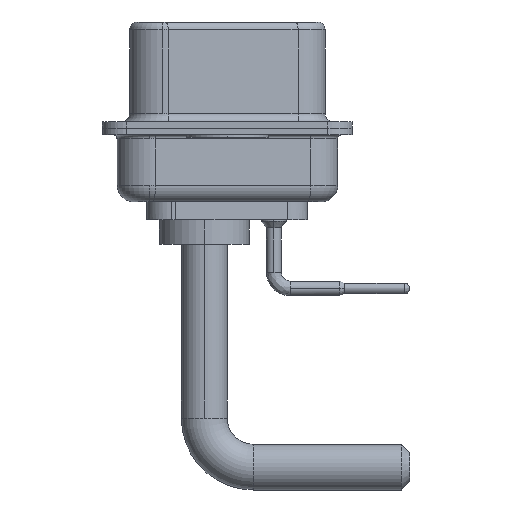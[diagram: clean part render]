
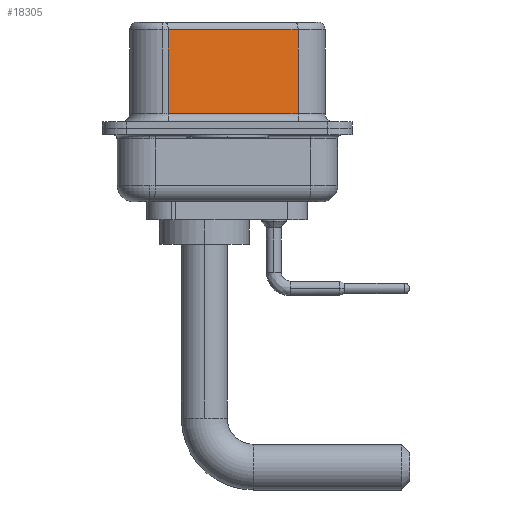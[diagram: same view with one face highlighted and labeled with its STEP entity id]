
A CAD part, left-side view. The second image highlights one B-rep face of the part: STEP entity #18305.
In plain terms, the highlighted planar face has unit normal (-0.985, -0.174, 0).
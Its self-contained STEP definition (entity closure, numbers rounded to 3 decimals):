
#445 = LINE ( 'NONE', #21000, #8310 ) ;
#653 = VERTEX_POINT ( 'NONE', #3463 ) ;
#831 = LINE ( 'NONE', #14577, #10171 ) ;
#2503 = EDGE_CURVE ( 'NONE', #653, #12462, #831, .T. ) ;
#3463 = CARTESIAN_POINT ( 'NONE',  ( 3.73, 3.628, 6.02 ) ) ;
#4261 = VECTOR ( 'NONE', #22033, 1000. ) ;
#5703 = ORIENTED_EDGE ( 'NONE', *, *, #13592, .F. ) ;
#5996 = VECTOR ( 'NONE', #9553, 1000. ) ;
#6199 = CARTESIAN_POINT ( 'NONE',  ( 5.132, -4.322, 6.52 ) ) ;
#6239 = VERTEX_POINT ( 'NONE', #21685 ) ;
#6333 = EDGE_LOOP ( 'NONE', ( #5703, #16460, #7844, #14801 ) ) ;
#6748 = CARTESIAN_POINT ( 'NONE',  ( 5.132, -4.322, 6.02 ) ) ;
#7844 = ORIENTED_EDGE ( 'NONE', *, *, #2503, .T. ) ;
#8310 = VECTOR ( 'NONE', #21101, 1000. ) ;
#9550 = VERTEX_POINT ( 'NONE', #12229 ) ;
#9553 = DIRECTION ( 'NONE',  ( 0., 0., -1. ) ) ;
#9778 = DIRECTION ( 'NONE',  ( -0.174, 0.985, 0. ) ) ;
#10171 = VECTOR ( 'NONE', #19817, 1000. ) ;
#10180 = LINE ( 'NONE', #6748, #4261 ) ;
#11218 = CARTESIAN_POINT ( 'NONE',  ( 5.132, -4.322, 6.52 ) ) ;
#11450 = FACE_OUTER_BOUND ( 'NONE', #6333, .T. ) ;
#12229 = CARTESIAN_POINT ( 'NONE',  ( 5.132, -4.322, 0.9 ) ) ;
#12462 = VERTEX_POINT ( 'NONE', #18582 ) ;
#13592 = EDGE_CURVE ( 'NONE', #6239, #9550, #21484, .T. ) ;
#14278 = DIRECTION ( 'NONE',  ( 0.985, 0.174, 0. ) ) ;
#14577 = CARTESIAN_POINT ( 'NONE',  ( 3.73, 3.628, 6.52 ) ) ;
#14612 = AXIS2_PLACEMENT_3D ( 'NONE', #11218, #14278, #9778 ) ;
#14801 = ORIENTED_EDGE ( 'NONE', *, *, #20710, .T. ) ;
#14916 = PLANE ( 'NONE',  #14612 ) ;
#16460 = ORIENTED_EDGE ( 'NONE', *, *, #17484, .T. ) ;
#17484 = EDGE_CURVE ( 'NONE', #6239, #653, #10180, .T. ) ;
#18305 = ADVANCED_FACE ( 'NONE', ( #11450 ), #14916, .F. ) ;
#18582 = CARTESIAN_POINT ( 'NONE',  ( 3.73, 3.628, 0.9 ) ) ;
#19817 = DIRECTION ( 'NONE',  ( 0., 0., -1. ) ) ;
#20710 = EDGE_CURVE ( 'NONE', #12462, #9550, #445, .T. ) ;
#21000 = CARTESIAN_POINT ( 'NONE',  ( 5.132, -4.322, 0.9 ) ) ;
#21101 = DIRECTION ( 'NONE',  ( 0.174, -0.985, 0. ) ) ;
#21484 = LINE ( 'NONE', #6199, #5996 ) ;
#21685 = CARTESIAN_POINT ( 'NONE',  ( 5.132, -4.322, 6.02 ) ) ;
#22033 = DIRECTION ( 'NONE',  ( -0.174, 0.985, 0. ) ) ;
